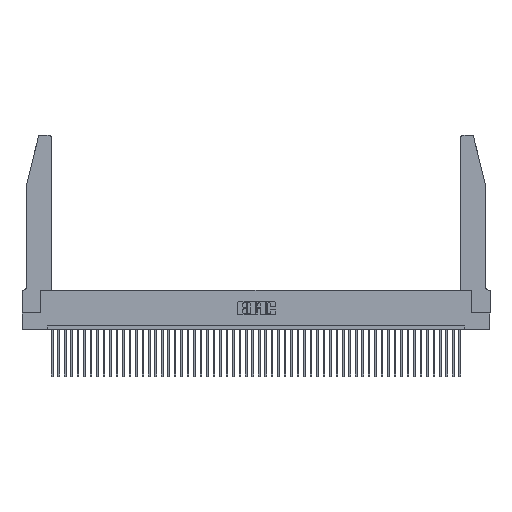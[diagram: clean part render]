
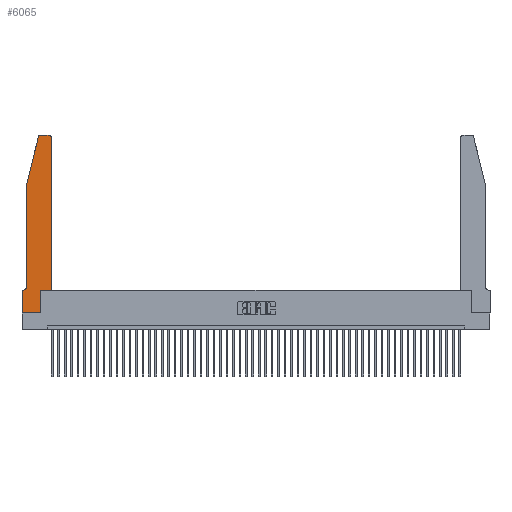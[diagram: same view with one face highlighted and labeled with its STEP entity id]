
A CAD part, top view. The second image highlights one B-rep face of the part: STEP entity #6065.
In plain terms, the highlighted planar face has unit normal (0, 0, 1).
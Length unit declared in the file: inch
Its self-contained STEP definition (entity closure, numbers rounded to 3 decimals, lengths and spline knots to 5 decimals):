
#324 = DIRECTION ( 'NONE',  ( 0., -1., 0. ) ) ;
#777 = EDGE_CURVE ( 'NONE', #6045, #49496, #13987, .T. ) ;
#1572 = DIRECTION ( 'NONE',  ( 1., 0., 0. ) ) ;
#1823 = VERTEX_POINT ( 'NONE', #46551 ) ;
#2999 = VECTOR ( 'NONE', #23827, 39.37008 ) ;
#3023 = CARTESIAN_POINT ( 'NONE',  ( 0., 0., 0.37 ) ) ;
#3728 = VECTOR ( 'NONE', #37489, 39.37008 ) ;
#3762 = VERTEX_POINT ( 'NONE', #23881 ) ;
#4305 = CARTESIAN_POINT ( 'NONE',  ( 0.2605, 2.75, 0.37 ) ) ;
#4465 = DIRECTION ( 'NONE',  ( 0., 0., -1. ) ) ;
#4647 = CARTESIAN_POINT ( 'NONE',  ( 0.0055, 0.42, 0.37 ) ) ;
#6045 = VERTEX_POINT ( 'NONE', #34120 ) ;
#6065 = ADVANCED_FACE ( 'NONE', ( #49156 ), #44101, .T. ) ;
#6510 = CARTESIAN_POINT ( 'NONE',  ( 0.4205, 2.75, 0.37 ) ) ;
#7130 = LINE ( 'NONE', #49375, #36705 ) ;
#7322 = VECTOR ( 'NONE', #25887, 39.37008 ) ;
#8455 = CARTESIAN_POINT ( 'NONE',  ( 0., 0., 0.37 ) ) ;
#8480 = EDGE_CURVE ( 'NONE', #25272, #1823, #18979, .T. ) ;
#9456 = CARTESIAN_POINT ( 'NONE',  ( 0.4205, 2.72, 0.37 ) ) ;
#10091 = VERTEX_POINT ( 'NONE', #28633 ) ;
#10306 = AXIS2_PLACEMENT_3D ( 'NONE', #32575, #36722, #44590 ) ;
#11224 = ORIENTED_EDGE ( 'NONE', *, *, #23293, .T. ) ;
#11653 = EDGE_CURVE ( 'NONE', #24914, #6045, #36610, .T. ) ;
#11839 = CARTESIAN_POINT ( 'NONE',  ( 0.2865, 0.35, 0.37 ) ) ;
#11898 = EDGE_CURVE ( 'NONE', #49896, #10091, #41367, .T. ) ;
#13202 = ORIENTED_EDGE ( 'NONE', *, *, #24581, .T. ) ;
#13321 = EDGE_LOOP ( 'NONE', ( #30028, #30664, #33859, #33879, #47099, #47696, #13202, #42257, #35424, #11224, #24469, #24330 ) ) ;
#13987 = CIRCLE ( 'NONE', #47275, 0.03 ) ;
#14377 = EDGE_CURVE ( 'NONE', #35024, #31050, #14577, .T. ) ;
#14577 = LINE ( 'NONE', #11839, #25535 ) ;
#15996 = EDGE_CURVE ( 'NONE', #33647, #35024, #27368, .T. ) ;
#16538 = DIRECTION ( 'NONE',  ( 1., 0., 0. ) ) ;
#17391 = CIRCLE ( 'NONE', #35614, 0.07 ) ;
#17952 = DIRECTION ( 'NONE',  ( 0., -1., 0. ) ) ;
#18810 = CARTESIAN_POINT ( 'NONE',  ( 0.0755, 2., 0.37 ) ) ;
#18979 = CIRCLE ( 'NONE', #35323, 0.03 ) ;
#21399 = VECTOR ( 'NONE', #31661, 39.37008 ) ;
#21595 = VECTOR ( 'NONE', #47152, 39.37008 ) ;
#23293 = EDGE_CURVE ( 'NONE', #31050, #24914, #33785, .T. ) ;
#23635 = EDGE_CURVE ( 'NONE', #36805, #3762, #26615, .T. ) ;
#23827 = DIRECTION ( 'NONE',  ( 1., 0., 0. ) ) ;
#23881 = CARTESIAN_POINT ( 'NONE',  ( 0.0755, 0.42, 0.37 ) ) ;
#24330 = ORIENTED_EDGE ( 'NONE', *, *, #777, .T. ) ;
#24469 = ORIENTED_EDGE ( 'NONE', *, *, #11653, .T. ) ;
#24581 = EDGE_CURVE ( 'NONE', #10091, #33647, #7130, .T. ) ;
#24914 = VERTEX_POINT ( 'NONE', #32406 ) ;
#25272 = VERTEX_POINT ( 'NONE', #31163 ) ;
#25535 = VECTOR ( 'NONE', #38606, 39.37008 ) ;
#25878 = CARTESIAN_POINT ( 'NONE',  ( 0.0755, 0.35, 0.37 ) ) ;
#25887 = DIRECTION ( 'NONE',  ( 1., 0., 0. ) ) ;
#26552 = EDGE_CURVE ( 'NONE', #49496, #25272, #38221, .T. ) ;
#26615 = LINE ( 'NONE', #37141, #28425 ) ;
#27368 = LINE ( 'NONE', #3023, #7322 ) ;
#28243 = VECTOR ( 'NONE', #33278, 39.37008 ) ;
#28425 = VECTOR ( 'NONE', #17952, 39.37008 ) ;
#28633 = CARTESIAN_POINT ( 'NONE',  ( 0., 0.35, 0.37 ) ) ;
#28999 = EDGE_CURVE ( 'NONE', #1823, #36805, #48343, .T. ) ;
#30028 = ORIENTED_EDGE ( 'NONE', *, *, #26552, .T. ) ;
#30664 = ORIENTED_EDGE ( 'NONE', *, *, #8480, .T. ) ;
#30893 = EDGE_CURVE ( 'NONE', #3762, #49896, #17391, .T. ) ;
#31050 = VERTEX_POINT ( 'NONE', #40509 ) ;
#31163 = CARTESIAN_POINT ( 'NONE',  ( 0.284, 2.75, 0.37 ) ) ;
#31661 = DIRECTION ( 'NONE',  ( -1., 0., 0. ) ) ;
#32406 = CARTESIAN_POINT ( 'NONE',  ( 0.4505, 0.35, 0.37 ) ) ;
#32575 = CARTESIAN_POINT ( 'NONE',  ( 0., 0.35, 0.37 ) ) ;
#33278 = DIRECTION ( 'NONE',  ( -1., 0., 0. ) ) ;
#33647 = VERTEX_POINT ( 'NONE', #8455 ) ;
#33707 = CARTESIAN_POINT ( 'NONE',  ( 0.0755, 2., 0.37 ) ) ;
#33785 = LINE ( 'NONE', #42751, #2999 ) ;
#33859 = ORIENTED_EDGE ( 'NONE', *, *, #28999, .T. ) ;
#33879 = ORIENTED_EDGE ( 'NONE', *, *, #23635, .T. ) ;
#34120 = CARTESIAN_POINT ( 'NONE',  ( 0.4505, 2.72, 0.37 ) ) ;
#35024 = VERTEX_POINT ( 'NONE', #44168 ) ;
#35323 = AXIS2_PLACEMENT_3D ( 'NONE', #43512, #35848, #1572 ) ;
#35424 = ORIENTED_EDGE ( 'NONE', *, *, #14377, .T. ) ;
#35541 = DIRECTION ( 'NONE',  ( -1., 0., 0. ) ) ;
#35614 = AXIS2_PLACEMENT_3D ( 'NONE', #4647, #4465, #35541 ) ;
#35848 = DIRECTION ( 'NONE',  ( 0., 0., 1. ) ) ;
#35863 = CARTESIAN_POINT ( 'NONE',  ( 0.0055, 0.35, 0.37 ) ) ;
#36610 = LINE ( 'NONE', #38249, #21595 ) ;
#36705 = VECTOR ( 'NONE', #324, 39.37008 ) ;
#36722 = DIRECTION ( 'NONE',  ( 0., 0., 1. ) ) ;
#36805 = VERTEX_POINT ( 'NONE', #33707 ) ;
#37141 = CARTESIAN_POINT ( 'NONE',  ( 0.0755, 2., 0.37 ) ) ;
#37489 = DIRECTION ( 'NONE',  ( -0.239, -0.971, 0. ) ) ;
#38221 = LINE ( 'NONE', #4305, #21399 ) ;
#38249 = CARTESIAN_POINT ( 'NONE',  ( 0.4505, 0.35, 0.37 ) ) ;
#38606 = DIRECTION ( 'NONE',  ( 0., 1., 0. ) ) ;
#39610 = DIRECTION ( 'NONE',  ( 0., 0., 1. ) ) ;
#40509 = CARTESIAN_POINT ( 'NONE',  ( 0.2865, 0.35, 0.37 ) ) ;
#41367 = LINE ( 'NONE', #25878, #28243 ) ;
#42257 = ORIENTED_EDGE ( 'NONE', *, *, #15996, .T. ) ;
#42751 = CARTESIAN_POINT ( 'NONE',  ( 0.4505, 0.35, 0.37 ) ) ;
#43512 = CARTESIAN_POINT ( 'NONE',  ( 0.284, 2.72, 0.37 ) ) ;
#44101 = PLANE ( 'NONE',  #10306 ) ;
#44168 = CARTESIAN_POINT ( 'NONE',  ( 0.2865, 0., 0.37 ) ) ;
#44590 = DIRECTION ( 'NONE',  ( 1., 0., 0. ) ) ;
#46551 = CARTESIAN_POINT ( 'NONE',  ( 0.25487, 2.72718, 0.37 ) ) ;
#47099 = ORIENTED_EDGE ( 'NONE', *, *, #30893, .T. ) ;
#47152 = DIRECTION ( 'NONE',  ( 0., 1., 0. ) ) ;
#47275 = AXIS2_PLACEMENT_3D ( 'NONE', #9456, #39610, #16538 ) ;
#47696 = ORIENTED_EDGE ( 'NONE', *, *, #11898, .T. ) ;
#48343 = LINE ( 'NONE', #18810, #3728 ) ;
#49156 = FACE_OUTER_BOUND ( 'NONE', #13321, .T. ) ;
#49375 = CARTESIAN_POINT ( 'NONE',  ( 0., 0., 0.37 ) ) ;
#49496 = VERTEX_POINT ( 'NONE', #6510 ) ;
#49896 = VERTEX_POINT ( 'NONE', #35863 ) ;
